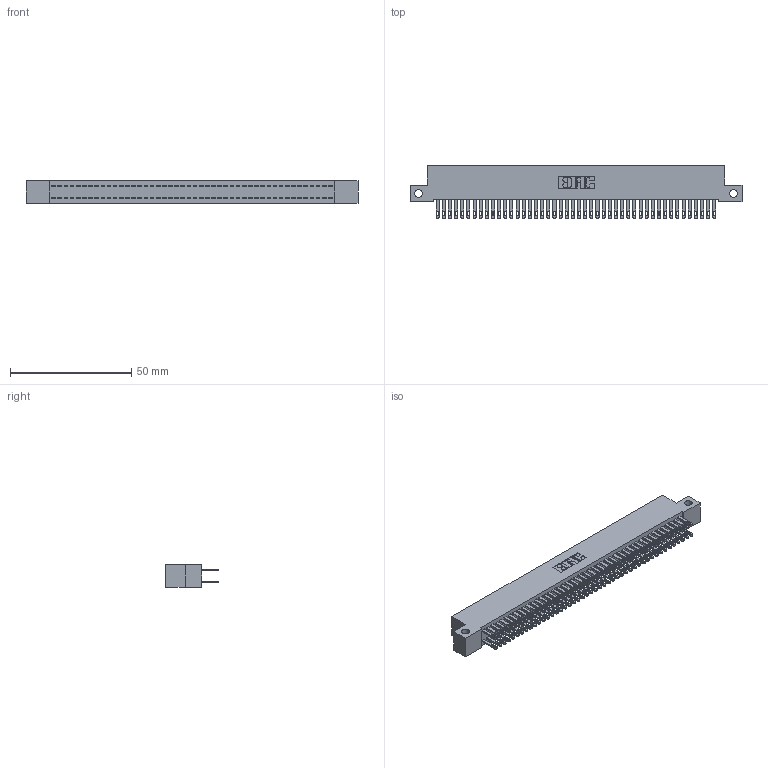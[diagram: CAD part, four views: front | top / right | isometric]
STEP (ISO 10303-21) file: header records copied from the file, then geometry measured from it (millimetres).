
FILE_DESCRIPTION (( 'STEP AP203' ), '1' );
FILE_NAME ('342-092-500-212.STEP', '2018-08-14T01:34:37', ( '' ), ( '' ), 'SwSTEP 2.0', 'SolidWorks 2016', '' );
FILE_SCHEMA (( 'CONFIG_CONTROL_DESIGN' ));
Length unit declared in the file: inch
Products named in the file (3): 342-092-500-212; 342 Part_Side Mount; 345-292-001_345-293-100
Assembly tree (93 placements, depth 2):
  342-092-500-212
    342 Part_Side Mount
    345-292-001_345-293-100  x92
Bounding box: 137.16 x 21.85 x 9.4 mm (x, y, z)
Volume: 12549.9 mm3; surface area: 21247.8 mm2
Topology: 93 solids, 93 shells, 4526 faces, 13823 edges, 9214 vertices
Faces by surface type: plane 2826, cylinder 1700
Entity records: 28877 total; most frequent: CARTESIAN_POINT 4778, ORIENTED_EDGE 4714, DIRECTION 4077, EDGE_CURVE 2357, LINE 2225, VECTOR 2225, VERTEX_POINT 1570, AXIS2_PLACEMENT_3D 926
